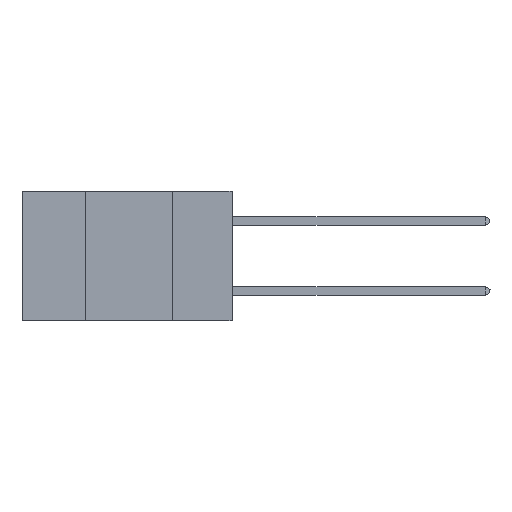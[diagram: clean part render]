
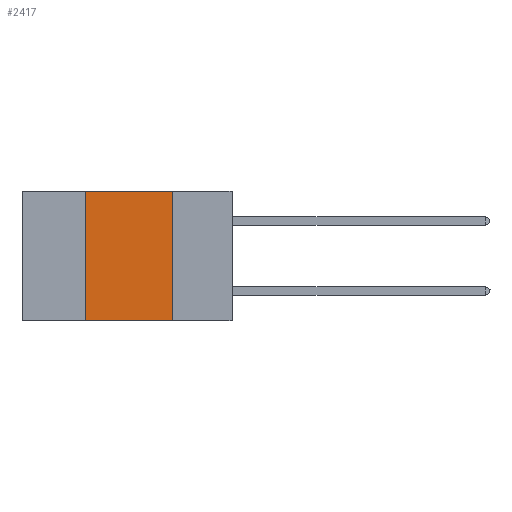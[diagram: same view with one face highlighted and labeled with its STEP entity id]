
A CAD part, left-side view. The second image highlights one B-rep face of the part: STEP entity #2417.
In plain terms, the highlighted planar face has unit normal (-1, 0, 0).
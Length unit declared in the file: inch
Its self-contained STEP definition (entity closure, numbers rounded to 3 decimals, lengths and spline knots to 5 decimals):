
#395 = EDGE_CURVE ( 'NONE', #30869, #14047, #21803, .T. ) ;
#612 = VERTEX_POINT ( 'NONE', #33810 ) ;
#2247 = LINE ( 'NONE', #16580, #12298 ) ;
#2417 = ADVANCED_FACE ( 'NONE', ( #29676 ), #24851, .F. ) ;
#3241 = DIRECTION ( 'NONE',  ( 1., 0., 0. ) ) ;
#9723 = CARTESIAN_POINT ( 'NONE',  ( 0., 0.6, 0. ) ) ;
#10421 = ORIENTED_EDGE ( 'NONE', *, *, #16992, .F. ) ;
#10682 = VERTEX_POINT ( 'NONE', #13000 ) ;
#11390 = CARTESIAN_POINT ( 'NONE',  ( 0., 0.6, 0. ) ) ;
#12016 = EDGE_LOOP ( 'NONE', ( #10421, #22009, #26955, #38042 ) ) ;
#12298 = VECTOR ( 'NONE', #19970, 39.37008 ) ;
#12641 = EDGE_CURVE ( 'NONE', #14047, #612, #41219, .T. ) ;
#13000 = CARTESIAN_POINT ( 'NONE',  ( 0., 0.17, -0.37 ) ) ;
#14047 = VERTEX_POINT ( 'NONE', #15044 ) ;
#14571 = DIRECTION ( 'NONE',  ( 0., -1., 0. ) ) ;
#15044 = CARTESIAN_POINT ( 'NONE',  ( 0., 0.42, 0. ) ) ;
#16580 = CARTESIAN_POINT ( 'NONE',  ( 0., 0.17, 0. ) ) ;
#16992 = EDGE_CURVE ( 'NONE', #612, #10682, #2247, .T. ) ;
#17200 = VECTOR ( 'NONE', #14571, 39.37008 ) ;
#18072 = EDGE_CURVE ( 'NONE', #30869, #10682, #22709, .T. ) ;
#19970 = DIRECTION ( 'NONE',  ( 0., 0., -1. ) ) ;
#20304 = VECTOR ( 'NONE', #32549, 39.37008 ) ;
#21407 = CARTESIAN_POINT ( 'NONE',  ( 0., 0.6, -0.37 ) ) ;
#21803 = LINE ( 'NONE', #29297, #20304 ) ;
#22009 = ORIENTED_EDGE ( 'NONE', *, *, #12641, .F. ) ;
#22709 = LINE ( 'NONE', #21407, #17200 ) ;
#24851 = PLANE ( 'NONE',  #34110 ) ;
#26955 = ORIENTED_EDGE ( 'NONE', *, *, #395, .F. ) ;
#29297 = CARTESIAN_POINT ( 'NONE',  ( 0., 0.42, 0. ) ) ;
#29676 = FACE_OUTER_BOUND ( 'NONE', #12016, .T. ) ;
#30869 = VERTEX_POINT ( 'NONE', #38870 ) ;
#31647 = VECTOR ( 'NONE', #33927, 39.37008 ) ;
#31959 = DIRECTION ( 'NONE',  ( 0., 0., -1. ) ) ;
#32549 = DIRECTION ( 'NONE',  ( 0., 0., 1. ) ) ;
#33810 = CARTESIAN_POINT ( 'NONE',  ( 0., 0.17, 0. ) ) ;
#33927 = DIRECTION ( 'NONE',  ( 0., -1., 0. ) ) ;
#34110 = AXIS2_PLACEMENT_3D ( 'NONE', #9723, #3241, #31959 ) ;
#38042 = ORIENTED_EDGE ( 'NONE', *, *, #18072, .T. ) ;
#38870 = CARTESIAN_POINT ( 'NONE',  ( 0., 0.42, -0.37 ) ) ;
#41219 = LINE ( 'NONE', #11390, #31647 ) ;
